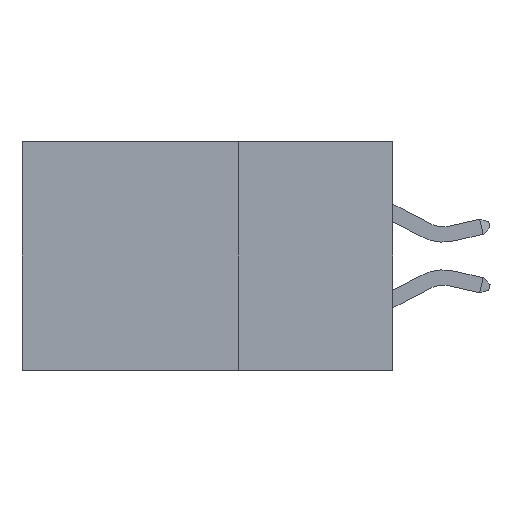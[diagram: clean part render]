
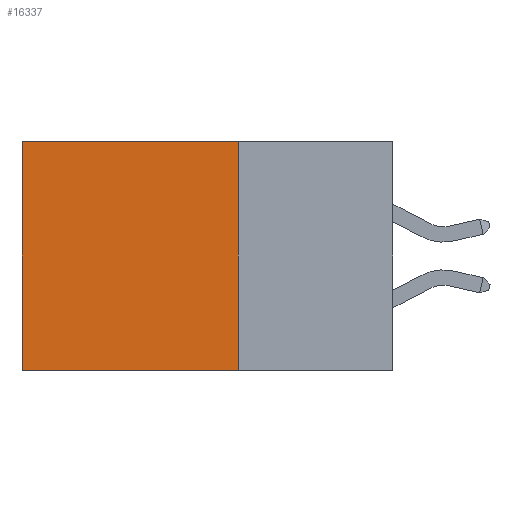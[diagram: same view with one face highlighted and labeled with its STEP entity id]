
A CAD part, left-side view. The second image highlights one B-rep face of the part: STEP entity #16337.
In plain terms, the highlighted planar face has unit normal (-1, 0, 0).
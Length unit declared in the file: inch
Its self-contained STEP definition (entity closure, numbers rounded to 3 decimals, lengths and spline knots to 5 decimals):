
#252 = LINE ( 'NONE', #17710, #3758 ) ;
#718 = AXIS2_PLACEMENT_3D ( 'NONE', #14229, #9896, #1158 ) ;
#1013 = VECTOR ( 'NONE', #14342, 39.37008 ) ;
#1158 = DIRECTION ( 'NONE',  ( 0., 0., -1. ) ) ;
#1205 = CARTESIAN_POINT ( 'NONE',  ( 0.2875, 0.6, 0. ) ) ;
#2297 = DIRECTION ( 'NONE',  ( 0., 1., 0. ) ) ;
#3758 = VECTOR ( 'NONE', #13514, 39.37008 ) ;
#4033 = VERTEX_POINT ( 'NONE', #7684 ) ;
#4586 = EDGE_LOOP ( 'NONE', ( #9536, #6433, #10890, #17732 ) ) ;
#5153 = EDGE_CURVE ( 'NONE', #5763, #5375, #13140, .T. ) ;
#5204 = VECTOR ( 'NONE', #10809, 39.37008 ) ;
#5375 = VERTEX_POINT ( 'NONE', #10468 ) ;
#5763 = VERTEX_POINT ( 'NONE', #9339 ) ;
#5787 = EDGE_CURVE ( 'NONE', #4033, #5375, #12876, .T. ) ;
#6433 = ORIENTED_EDGE ( 'NONE', *, *, #5787, .F. ) ;
#6767 = EDGE_CURVE ( 'NONE', #9436, #4033, #252, .T. ) ;
#7684 = CARTESIAN_POINT ( 'NONE',  ( 0.2875, 0.25, -0.37 ) ) ;
#8479 = PLANE ( 'NONE',  #718 ) ;
#9339 = CARTESIAN_POINT ( 'NONE',  ( 0.2875, 0.6, 0. ) ) ;
#9436 = VERTEX_POINT ( 'NONE', #15289 ) ;
#9476 = CARTESIAN_POINT ( 'NONE',  ( 0.2875, 0.25, 0. ) ) ;
#9536 = ORIENTED_EDGE ( 'NONE', *, *, #5153, .T. ) ;
#9896 = DIRECTION ( 'NONE',  ( 1., 0., 0. ) ) ;
#10468 = CARTESIAN_POINT ( 'NONE',  ( 0.2875, 0.6, -0.37 ) ) ;
#10809 = DIRECTION ( 'NONE',  ( 0., 1., 0. ) ) ;
#10890 = ORIENTED_EDGE ( 'NONE', *, *, #6767, .F. ) ;
#12876 = LINE ( 'NONE', #16597, #5204 ) ;
#12950 = FACE_OUTER_BOUND ( 'NONE', #4586, .T. ) ;
#13140 = LINE ( 'NONE', #1205, #1013 ) ;
#13514 = DIRECTION ( 'NONE',  ( 0., 0., -1. ) ) ;
#14229 = CARTESIAN_POINT ( 'NONE',  ( 0.2875, 0.25, 0. ) ) ;
#14342 = DIRECTION ( 'NONE',  ( 0., 0., -1. ) ) ;
#14510 = VECTOR ( 'NONE', #2297, 39.37008 ) ;
#15289 = CARTESIAN_POINT ( 'NONE',  ( 0.2875, 0.25, 0. ) ) ;
#16187 = EDGE_CURVE ( 'NONE', #9436, #5763, #18246, .T. ) ;
#16337 = ADVANCED_FACE ( 'NONE', ( #12950 ), #8479, .F. ) ;
#16597 = CARTESIAN_POINT ( 'NONE',  ( 0.2875, 0.25, -0.37 ) ) ;
#17710 = CARTESIAN_POINT ( 'NONE',  ( 0.2875, 0.25, 0. ) ) ;
#17732 = ORIENTED_EDGE ( 'NONE', *, *, #16187, .T. ) ;
#18246 = LINE ( 'NONE', #9476, #14510 ) ;
